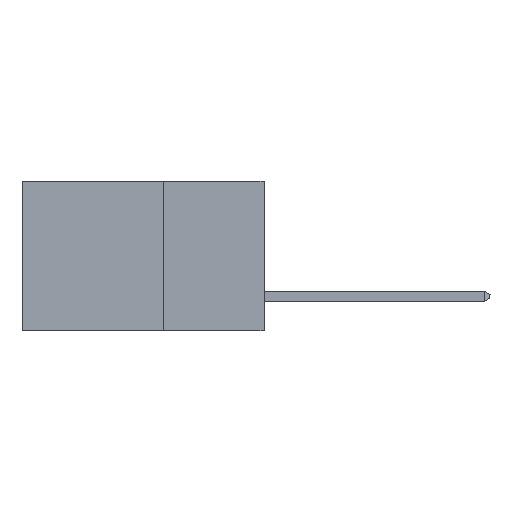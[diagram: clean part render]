
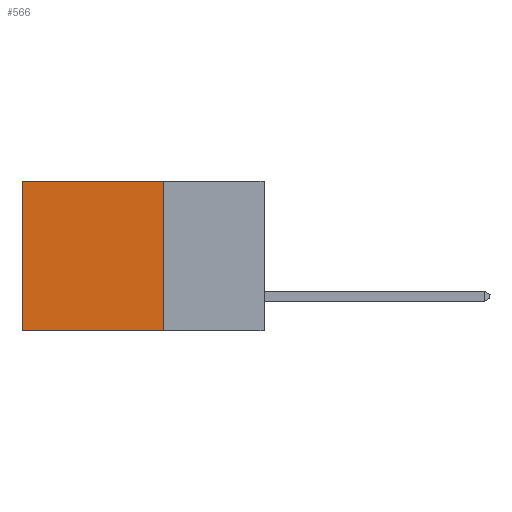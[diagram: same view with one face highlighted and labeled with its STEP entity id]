
A CAD part, left-side view. The second image highlights one B-rep face of the part: STEP entity #566.
In plain terms, the highlighted planar face has unit normal (-1, 0, 0).
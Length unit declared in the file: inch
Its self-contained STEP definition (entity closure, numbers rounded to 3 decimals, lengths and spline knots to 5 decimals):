
#435 = FACE_OUTER_BOUND ( 'NONE', #3393, .T. ) ;
#566 = ADVANCED_FACE ( 'NONE', ( #435 ), #10884, .F. ) ;
#1035 = CARTESIAN_POINT ( 'NONE',  ( 0.2615, 0.6, -0.37 ) ) ;
#2403 = DIRECTION ( 'NONE',  ( 1., 0., 0. ) ) ;
#2581 = VECTOR ( 'NONE', #3524, 39.37008 ) ;
#3296 = DIRECTION ( 'NONE',  ( 0., 0., -1. ) ) ;
#3393 = EDGE_LOOP ( 'NONE', ( #10542, #9238, #11599, #7527 ) ) ;
#3524 = DIRECTION ( 'NONE',  ( 0., 0., -1. ) ) ;
#4110 = EDGE_CURVE ( 'NONE', #13374, #14378, #7614, .T. ) ;
#4326 = CARTESIAN_POINT ( 'NONE',  ( 0.2615, 0.25, -0.37 ) ) ;
#4465 = CARTESIAN_POINT ( 'NONE',  ( 0.2615, 0.25, -0.37 ) ) ;
#4617 = CARTESIAN_POINT ( 'NONE',  ( 0.2615, 0.6, -0.37 ) ) ;
#5373 = DIRECTION ( 'NONE',  ( 0., 1., 0. ) ) ;
#5386 = VECTOR ( 'NONE', #5373, 39.37008 ) ;
#5934 = VECTOR ( 'NONE', #11547, 39.37008 ) ;
#6243 = CARTESIAN_POINT ( 'NONE',  ( 0.2615, 0.6, 0. ) ) ;
#7527 = ORIENTED_EDGE ( 'NONE', *, *, #15072, .T. ) ;
#7614 = LINE ( 'NONE', #15323, #2581 ) ;
#8000 = LINE ( 'NONE', #9037, #5386 ) ;
#8231 = AXIS2_PLACEMENT_3D ( 'NONE', #4326, #2403, #3296 ) ;
#9037 = CARTESIAN_POINT ( 'NONE',  ( 0.2615, 0.25, 0. ) ) ;
#9238 = ORIENTED_EDGE ( 'NONE', *, *, #14125, .F. ) ;
#10408 = CARTESIAN_POINT ( 'NONE',  ( 0.2615, 0.25, 0. ) ) ;
#10542 = ORIENTED_EDGE ( 'NONE', *, *, #14792, .T. ) ;
#10884 = PLANE ( 'NONE',  #8231 ) ;
#11170 = LINE ( 'NONE', #4617, #14459 ) ;
#11505 = VERTEX_POINT ( 'NONE', #6243 ) ;
#11547 = DIRECTION ( 'NONE',  ( 0., 1., 0. ) ) ;
#11599 = ORIENTED_EDGE ( 'NONE', *, *, #4110, .F. ) ;
#11631 = LINE ( 'NONE', #12920, #5934 ) ;
#12920 = CARTESIAN_POINT ( 'NONE',  ( 0.2615, 0.25, -0.37 ) ) ;
#13374 = VERTEX_POINT ( 'NONE', #10408 ) ;
#13582 = DIRECTION ( 'NONE',  ( 0., 0., -1. ) ) ;
#14125 = EDGE_CURVE ( 'NONE', #14378, #15462, #11631, .T. ) ;
#14378 = VERTEX_POINT ( 'NONE', #4465 ) ;
#14459 = VECTOR ( 'NONE', #13582, 39.37008 ) ;
#14792 = EDGE_CURVE ( 'NONE', #11505, #15462, #11170, .T. ) ;
#15072 = EDGE_CURVE ( 'NONE', #13374, #11505, #8000, .T. ) ;
#15323 = CARTESIAN_POINT ( 'NONE',  ( 0.2615, 0.25, -0.37 ) ) ;
#15462 = VERTEX_POINT ( 'NONE', #1035 ) ;
